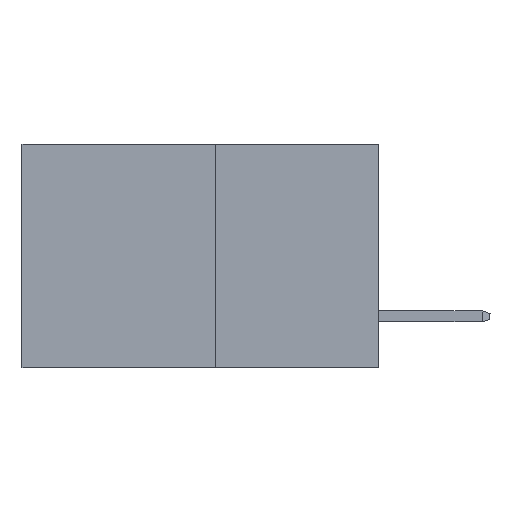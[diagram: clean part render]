
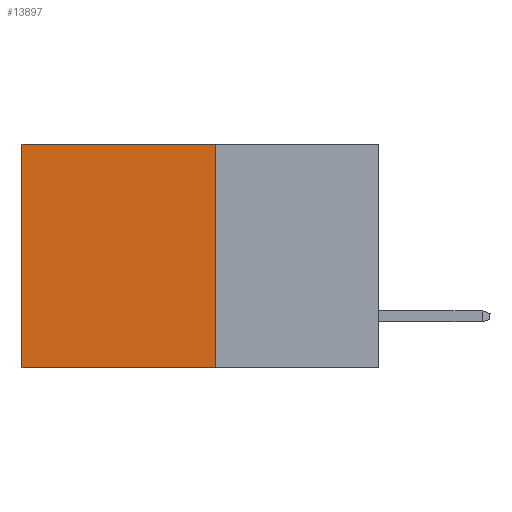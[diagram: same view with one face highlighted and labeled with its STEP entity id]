
A CAD part, left-side view. The second image highlights one B-rep face of the part: STEP entity #13897.
In plain terms, the highlighted planar face has unit normal (-1, 0, 0).
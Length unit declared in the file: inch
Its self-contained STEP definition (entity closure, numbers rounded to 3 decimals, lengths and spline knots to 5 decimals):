
#123 = CARTESIAN_POINT ( 'NONE',  ( 0.277, 0.59, -0.37 ) ) ;
#713 = VECTOR ( 'NONE', #8340, 39.37008 ) ;
#758 = EDGE_CURVE ( 'NONE', #16635, #12756, #8498, .T. ) ;
#1599 = DIRECTION ( 'NONE',  ( 0., 0., -1. ) ) ;
#2935 = LINE ( 'NONE', #123, #6382 ) ;
#4242 = CARTESIAN_POINT ( 'NONE',  ( 0.277, 0.27, -0.37 ) ) ;
#4455 = VERTEX_POINT ( 'NONE', #15242 ) ;
#4800 = LINE ( 'NONE', #8355, #9206 ) ;
#5847 = FACE_OUTER_BOUND ( 'NONE', #14050, .T. ) ;
#6116 = EDGE_CURVE ( 'NONE', #17311, #4455, #4800, .T. ) ;
#6382 = VECTOR ( 'NONE', #1599, 39.37008 ) ;
#6827 = PLANE ( 'NONE',  #12038 ) ;
#6933 = CARTESIAN_POINT ( 'NONE',  ( 0.277, 0.59, -0.37 ) ) ;
#7129 = ORIENTED_EDGE ( 'NONE', *, *, #758, .F. ) ;
#7937 = DIRECTION ( 'NONE',  ( 0., 0., -1. ) ) ;
#8340 = DIRECTION ( 'NONE',  ( 0., 1., 0. ) ) ;
#8355 = CARTESIAN_POINT ( 'NONE',  ( 0.277, 0.27, 0. ) ) ;
#8498 = LINE ( 'NONE', #10932, #713 ) ;
#9206 = VECTOR ( 'NONE', #9359, 39.37008 ) ;
#9359 = DIRECTION ( 'NONE',  ( 0., 1., 0. ) ) ;
#9781 = DIRECTION ( 'NONE',  ( 0., 0., -1. ) ) ;
#10559 = ORIENTED_EDGE ( 'NONE', *, *, #17946, .T. ) ;
#10932 = CARTESIAN_POINT ( 'NONE',  ( 0.277, 0.27, -0.37 ) ) ;
#11464 = ORIENTED_EDGE ( 'NONE', *, *, #11931, .F. ) ;
#11931 = EDGE_CURVE ( 'NONE', #17311, #16635, #16742, .T. ) ;
#12038 = AXIS2_PLACEMENT_3D ( 'NONE', #17012, #18455, #9781 ) ;
#12242 = CARTESIAN_POINT ( 'NONE',  ( 0.277, 0.27, -0.37 ) ) ;
#12756 = VERTEX_POINT ( 'NONE', #6933 ) ;
#12956 = CARTESIAN_POINT ( 'NONE',  ( 0.277, 0.27, 0. ) ) ;
#13301 = VECTOR ( 'NONE', #7937, 39.37008 ) ;
#13897 = ADVANCED_FACE ( 'NONE', ( #5847 ), #6827, .F. ) ;
#14050 = EDGE_LOOP ( 'NONE', ( #10559, #7129, #11464, #15310 ) ) ;
#15242 = CARTESIAN_POINT ( 'NONE',  ( 0.277, 0.59, 0. ) ) ;
#15310 = ORIENTED_EDGE ( 'NONE', *, *, #6116, .T. ) ;
#16635 = VERTEX_POINT ( 'NONE', #4242 ) ;
#16742 = LINE ( 'NONE', #12242, #13301 ) ;
#17012 = CARTESIAN_POINT ( 'NONE',  ( 0.277, 0.27, -0.37 ) ) ;
#17311 = VERTEX_POINT ( 'NONE', #12956 ) ;
#17946 = EDGE_CURVE ( 'NONE', #4455, #12756, #2935, .T. ) ;
#18455 = DIRECTION ( 'NONE',  ( 1., 0., 0. ) ) ;
